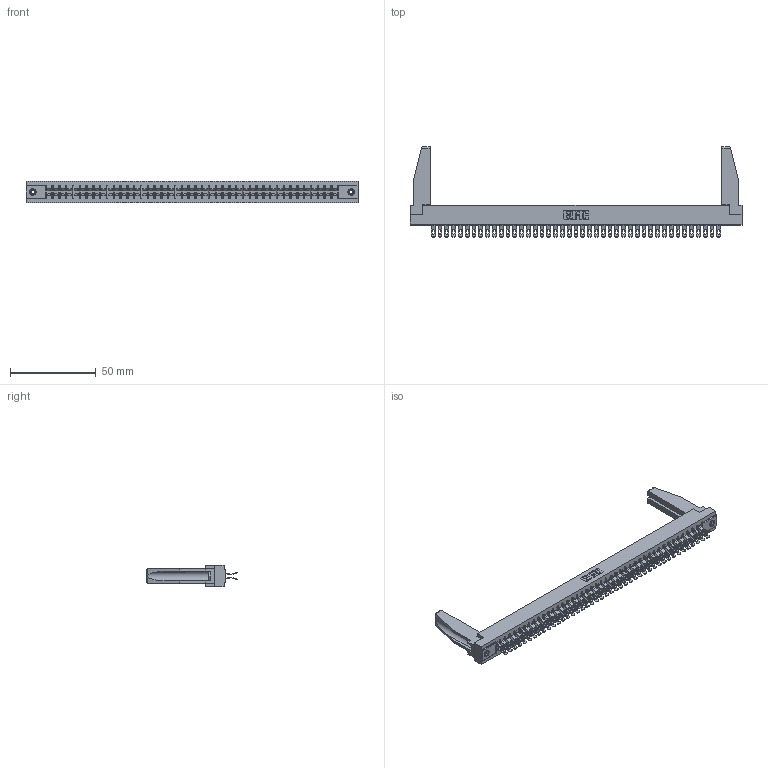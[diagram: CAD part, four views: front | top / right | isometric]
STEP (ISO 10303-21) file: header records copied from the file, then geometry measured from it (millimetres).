
FILE_DESCRIPTION (( 'STEP AP203' ), '1' );
FILE_NAME ('355-086-555-578.STEP', '2019-09-13T16:59:06', ( '' ), ( '' ), 'SwSTEP 2.0', 'SolidWorks 2016', '' );
FILE_SCHEMA (( 'CONFIG_CONTROL_DESIGN' ));
Length unit declared in the file: inch
Products named in the file (5): 305-290-001_555; 305 Part_.156 Dia; 345-250-001_345-250-001-102; 355-086-555-578; 307-220-078
Assembly tree (91 placements, depth 2):
  355-086-555-578
    305 Part_.156 Dia
    305-290-001_555  x86
    345-250-001_345-250-001-102  x2
    307-220-078  x2
Bounding box: 193.4 x 52.45 x 12.7 mm (x, y, z)
Volume: 23835.3 mm3; surface area: 31662.8 mm2
Topology: 91 solids, 91 shells, 5922 faces, 17631 edges, 11514 vertices
Faces by surface type: plane 2904, cylinder 2830, sphere 172, cone 12, torus 4
Entity records: 49499 total; most frequent: CARTESIAN_POINT 8215, ORIENTED_EDGE 8104, DIRECTION 7898, EDGE_CURVE 4052, VECTOR 3256, LINE 3256, VERTEX_POINT 2580, AXIS2_PLACEMENT_3D 2321
